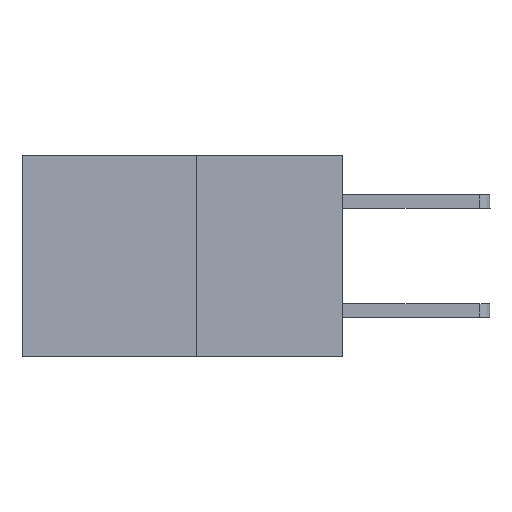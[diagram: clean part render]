
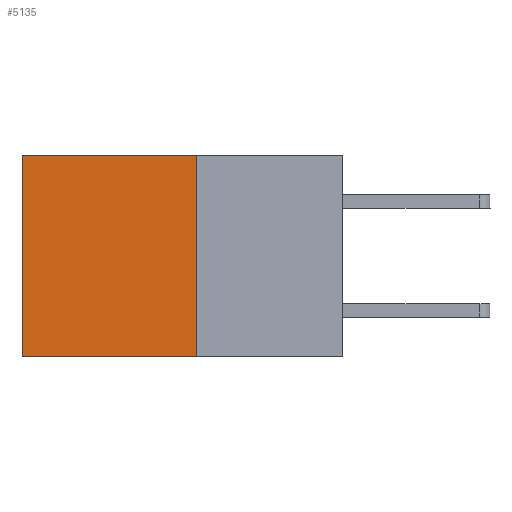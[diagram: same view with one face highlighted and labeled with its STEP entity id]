
A CAD part, left-side view. The second image highlights one B-rep face of the part: STEP entity #5135.
In plain terms, the highlighted planar face has unit normal (-1, 0, 0).
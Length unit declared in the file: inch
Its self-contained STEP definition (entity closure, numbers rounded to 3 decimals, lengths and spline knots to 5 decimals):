
#45 = DIRECTION ( 'NONE',  ( 0., 1., 0. ) ) ;
#141 = VERTEX_POINT ( 'NONE', #4874 ) ;
#995 = PLANE ( 'NONE',  #3588 ) ;
#998 = LINE ( 'NONE', #3391, #2704 ) ;
#1057 = CARTESIAN_POINT ( 'NONE',  ( 0.277, 0.27, -0.37 ) ) ;
#1358 = LINE ( 'NONE', #1950, #6384 ) ;
#1494 = VECTOR ( 'NONE', #2667, 39.37008 ) ;
#1723 = VERTEX_POINT ( 'NONE', #5434 ) ;
#1950 = CARTESIAN_POINT ( 'NONE',  ( 0.277, 0.59, -0.37 ) ) ;
#2161 = EDGE_CURVE ( 'NONE', #4336, #1723, #998, .T. ) ;
#2667 = DIRECTION ( 'NONE',  ( 0., 0., -1. ) ) ;
#2704 = VECTOR ( 'NONE', #45, 39.37008 ) ;
#3041 = DIRECTION ( 'NONE',  ( 0., 0., -1. ) ) ;
#3221 = EDGE_CURVE ( 'NONE', #4336, #7591, #8082, .T. ) ;
#3391 = CARTESIAN_POINT ( 'NONE',  ( 0.277, 0.27, 0. ) ) ;
#3588 = AXIS2_PLACEMENT_3D ( 'NONE', #1057, #6206, #6069 ) ;
#3898 = ORIENTED_EDGE ( 'NONE', *, *, #3221, .F. ) ;
#3958 = ORIENTED_EDGE ( 'NONE', *, *, #4139, .T. ) ;
#4139 = EDGE_CURVE ( 'NONE', #1723, #141, #1358, .T. ) ;
#4193 = CARTESIAN_POINT ( 'NONE',  ( 0.277, 0.27, 0. ) ) ;
#4336 = VERTEX_POINT ( 'NONE', #4193 ) ;
#4726 = CARTESIAN_POINT ( 'NONE',  ( 0.277, 0.27, -0.37 ) ) ;
#4864 = CARTESIAN_POINT ( 'NONE',  ( 0.277, 0.27, -0.37 ) ) ;
#4874 = CARTESIAN_POINT ( 'NONE',  ( 0.277, 0.59, -0.37 ) ) ;
#5135 = ADVANCED_FACE ( 'NONE', ( #6365 ), #995, .F. ) ;
#5434 = CARTESIAN_POINT ( 'NONE',  ( 0.277, 0.59, 0. ) ) ;
#5564 = DIRECTION ( 'NONE',  ( 0., 1., 0. ) ) ;
#6069 = DIRECTION ( 'NONE',  ( 0., 0., -1. ) ) ;
#6206 = DIRECTION ( 'NONE',  ( 1., 0., 0. ) ) ;
#6365 = FACE_OUTER_BOUND ( 'NONE', #7543, .T. ) ;
#6384 = VECTOR ( 'NONE', #3041, 39.37008 ) ;
#6733 = LINE ( 'NONE', #4864, #7955 ) ;
#6768 = ORIENTED_EDGE ( 'NONE', *, *, #8208, .F. ) ;
#7343 = CARTESIAN_POINT ( 'NONE',  ( 0.277, 0.27, -0.37 ) ) ;
#7518 = ORIENTED_EDGE ( 'NONE', *, *, #2161, .T. ) ;
#7543 = EDGE_LOOP ( 'NONE', ( #3958, #6768, #3898, #7518 ) ) ;
#7591 = VERTEX_POINT ( 'NONE', #7343 ) ;
#7955 = VECTOR ( 'NONE', #5564, 39.37008 ) ;
#8082 = LINE ( 'NONE', #4726, #1494 ) ;
#8208 = EDGE_CURVE ( 'NONE', #7591, #141, #6733, .T. ) ;
